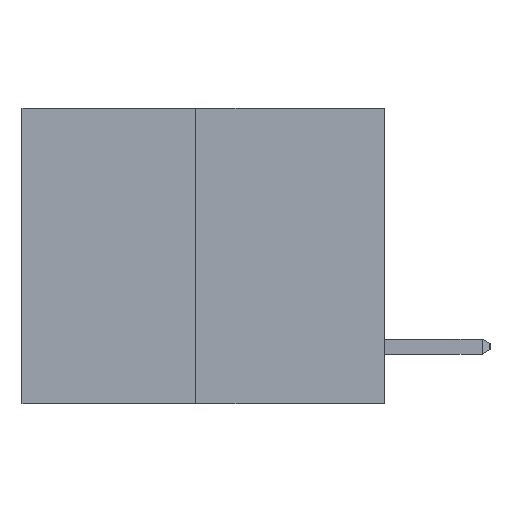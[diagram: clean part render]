
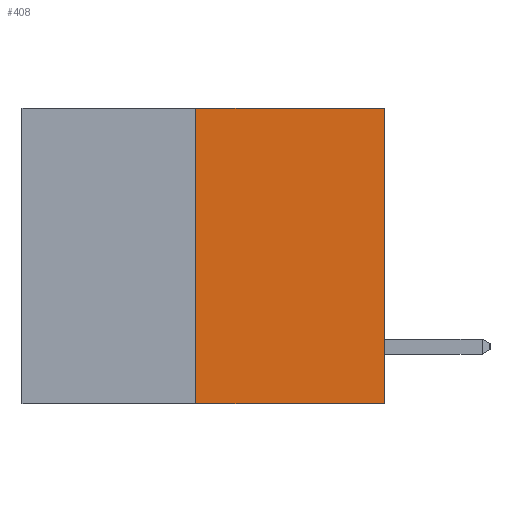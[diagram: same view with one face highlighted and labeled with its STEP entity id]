
A CAD part, left-side view. The second image highlights one B-rep face of the part: STEP entity #408.
In plain terms, the highlighted planar face has unit normal (-1, 0, 0).
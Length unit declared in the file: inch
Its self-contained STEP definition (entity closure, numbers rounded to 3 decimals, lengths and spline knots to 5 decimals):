
#182 = CARTESIAN_POINT ( 'NONE',  ( 0., 0.6, 0. ) ) ;
#408 = ADVANCED_FACE ( 'NONE', ( #2267 ), #2240, .F. ) ;
#431 = EDGE_CURVE ( 'NONE', #9352, #6021, #13397, .T. ) ;
#1780 = VECTOR ( 'NONE', #2203, 39.37008 ) ;
#2173 = EDGE_CURVE ( 'NONE', #9352, #11084, #3819, .T. ) ;
#2203 = DIRECTION ( 'NONE',  ( 0., -1., 0. ) ) ;
#2240 = PLANE ( 'NONE',  #9475 ) ;
#2267 = FACE_OUTER_BOUND ( 'NONE', #3389, .T. ) ;
#2613 = ORIENTED_EDGE ( 'NONE', *, *, #6969, .T. ) ;
#3389 = EDGE_LOOP ( 'NONE', ( #5230, #9826, #2613, #11713 ) ) ;
#3748 = LINE ( 'NONE', #7945, #9064 ) ;
#3819 = LINE ( 'NONE', #8076, #11728 ) ;
#5230 = ORIENTED_EDGE ( 'NONE', *, *, #431, .F. ) ;
#5818 = VECTOR ( 'NONE', #6388, 39.37008 ) ;
#6021 = VERTEX_POINT ( 'NONE', #8180 ) ;
#6052 = CARTESIAN_POINT ( 'NONE',  ( 0., 0., 0. ) ) ;
#6388 = DIRECTION ( 'NONE',  ( 0., 0., 1. ) ) ;
#6969 = EDGE_CURVE ( 'NONE', #11084, #7102, #3748, .T. ) ;
#7102 = VERTEX_POINT ( 'NONE', #6052 ) ;
#7914 = LINE ( 'NONE', #8426, #1780 ) ;
#7945 = CARTESIAN_POINT ( 'NONE',  ( 0., 0., 0. ) ) ;
#8076 = CARTESIAN_POINT ( 'NONE',  ( 0., 0.6, -0.49 ) ) ;
#8180 = CARTESIAN_POINT ( 'NONE',  ( 0., 0.312, 0. ) ) ;
#8426 = CARTESIAN_POINT ( 'NONE',  ( 0., 0.6, 0. ) ) ;
#9064 = VECTOR ( 'NONE', #10063, 39.37008 ) ;
#9315 = DIRECTION ( 'NONE',  ( 0., 0., -1. ) ) ;
#9352 = VERTEX_POINT ( 'NONE', #12385 ) ;
#9475 = AXIS2_PLACEMENT_3D ( 'NONE', #182, #10397, #9315 ) ;
#9826 = ORIENTED_EDGE ( 'NONE', *, *, #2173, .T. ) ;
#10063 = DIRECTION ( 'NONE',  ( 0., 0., 1. ) ) ;
#10147 = DIRECTION ( 'NONE',  ( 0., -1., 0. ) ) ;
#10397 = DIRECTION ( 'NONE',  ( 1., 0., 0. ) ) ;
#10449 = CARTESIAN_POINT ( 'NONE',  ( 0., 0.312, -0.49 ) ) ;
#11084 = VERTEX_POINT ( 'NONE', #13257 ) ;
#11713 = ORIENTED_EDGE ( 'NONE', *, *, #12049, .F. ) ;
#11728 = VECTOR ( 'NONE', #10147, 39.37008 ) ;
#12049 = EDGE_CURVE ( 'NONE', #6021, #7102, #7914, .T. ) ;
#12385 = CARTESIAN_POINT ( 'NONE',  ( 0., 0.312, -0.49 ) ) ;
#13257 = CARTESIAN_POINT ( 'NONE',  ( 0., 0., -0.49 ) ) ;
#13397 = LINE ( 'NONE', #10449, #5818 ) ;
